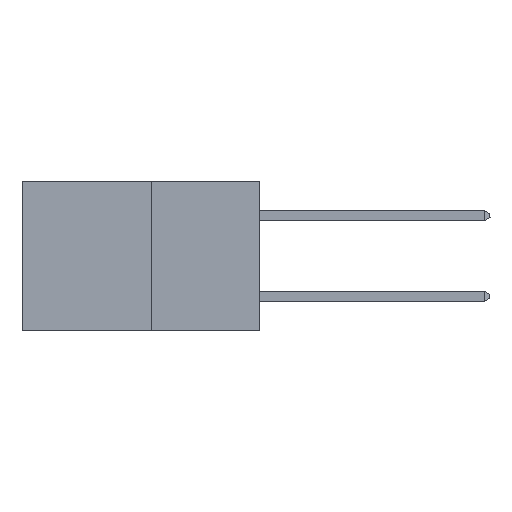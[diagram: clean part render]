
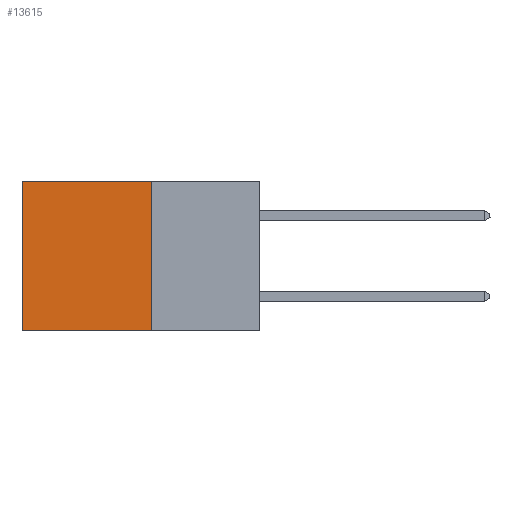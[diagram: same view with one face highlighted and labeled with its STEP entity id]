
A CAD part, left-side view. The second image highlights one B-rep face of the part: STEP entity #13615.
In plain terms, the highlighted planar face has unit normal (-1, 0, 0).
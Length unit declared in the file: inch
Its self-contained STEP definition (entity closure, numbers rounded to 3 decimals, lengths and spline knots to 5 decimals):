
#452 = VECTOR ( 'NONE', #17944, 39.37008 ) ;
#2537 = LINE ( 'NONE', #13254, #2987 ) ;
#2987 = VECTOR ( 'NONE', #12944, 39.37008 ) ;
#3010 = EDGE_CURVE ( 'NONE', #13432, #3114, #2537, .T. ) ;
#3114 = VERTEX_POINT ( 'NONE', #8725 ) ;
#3473 = EDGE_CURVE ( 'NONE', #5576, #11938, #13448, .T. ) ;
#3972 = DIRECTION ( 'NONE',  ( 0., 0., -1. ) ) ;
#5576 = VERTEX_POINT ( 'NONE', #17044 ) ;
#5895 = VECTOR ( 'NONE', #12715, 39.37008 ) ;
#7117 = LINE ( 'NONE', #15862, #14186 ) ;
#7813 = CARTESIAN_POINT ( 'NONE',  ( 0.277, 0.59, -0.37 ) ) ;
#8339 = ORIENTED_EDGE ( 'NONE', *, *, #3010, .T. ) ;
#8420 = ORIENTED_EDGE ( 'NONE', *, *, #14291, .T. ) ;
#8725 = CARTESIAN_POINT ( 'NONE',  ( 0.277, 0.59, 0. ) ) ;
#8784 = FACE_OUTER_BOUND ( 'NONE', #17067, .T. ) ;
#9663 = PLANE ( 'NONE',  #11385 ) ;
#10634 = CARTESIAN_POINT ( 'NONE',  ( 0.277, 0.27, 0. ) ) ;
#10985 = CARTESIAN_POINT ( 'NONE',  ( 0.277, 0.59, -0.37 ) ) ;
#11385 = AXIS2_PLACEMENT_3D ( 'NONE', #16694, #12505, #3972 ) ;
#11418 = LINE ( 'NONE', #10985, #452 ) ;
#11746 = EDGE_CURVE ( 'NONE', #13432, #5576, #7117, .T. ) ;
#11938 = VERTEX_POINT ( 'NONE', #7813 ) ;
#12409 = ORIENTED_EDGE ( 'NONE', *, *, #3473, .F. ) ;
#12505 = DIRECTION ( 'NONE',  ( 1., 0., 0. ) ) ;
#12715 = DIRECTION ( 'NONE',  ( 0., 1., 0. ) ) ;
#12944 = DIRECTION ( 'NONE',  ( 0., 1., 0. ) ) ;
#13254 = CARTESIAN_POINT ( 'NONE',  ( 0.277, 0.27, 0. ) ) ;
#13432 = VERTEX_POINT ( 'NONE', #10634 ) ;
#13448 = LINE ( 'NONE', #15251, #5895 ) ;
#13609 = ORIENTED_EDGE ( 'NONE', *, *, #11746, .F. ) ;
#13615 = ADVANCED_FACE ( 'NONE', ( #8784 ), #9663, .F. ) ;
#14186 = VECTOR ( 'NONE', #17215, 39.37008 ) ;
#14291 = EDGE_CURVE ( 'NONE', #3114, #11938, #11418, .T. ) ;
#15251 = CARTESIAN_POINT ( 'NONE',  ( 0.277, 0.27, -0.37 ) ) ;
#15862 = CARTESIAN_POINT ( 'NONE',  ( 0.277, 0.27, -0.37 ) ) ;
#16694 = CARTESIAN_POINT ( 'NONE',  ( 0.277, 0.27, -0.37 ) ) ;
#17044 = CARTESIAN_POINT ( 'NONE',  ( 0.277, 0.27, -0.37 ) ) ;
#17067 = EDGE_LOOP ( 'NONE', ( #8420, #12409, #13609, #8339 ) ) ;
#17215 = DIRECTION ( 'NONE',  ( 0., 0., -1. ) ) ;
#17944 = DIRECTION ( 'NONE',  ( 0., 0., -1. ) ) ;
